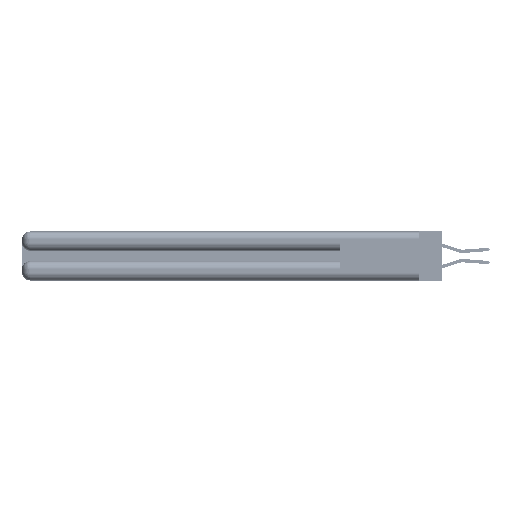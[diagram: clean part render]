
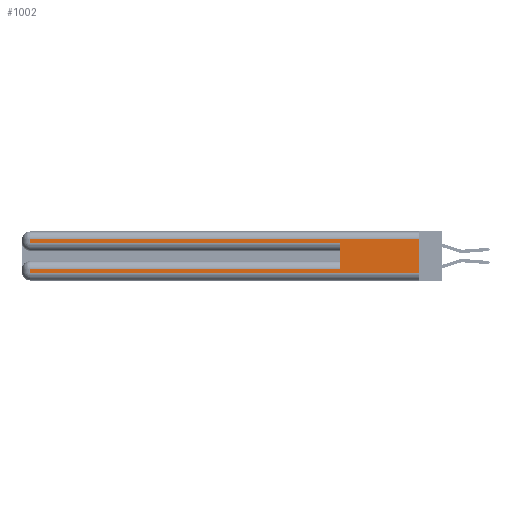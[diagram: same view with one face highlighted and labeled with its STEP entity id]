
A CAD part, left-side view. The second image highlights one B-rep face of the part: STEP entity #1002.
In plain terms, the highlighted planar face has unit normal (-1, 0, 0).
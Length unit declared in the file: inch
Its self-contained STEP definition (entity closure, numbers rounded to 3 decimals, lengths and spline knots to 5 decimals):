
#523 = VERTEX_POINT ( 'NONE', #30071 ) ;
#1002 = ADVANCED_FACE ( 'NONE', ( #9338 ), #17285, .F. ) ;
#1548 = LINE ( 'NONE', #7490, #26952 ) ;
#1995 = VERTEX_POINT ( 'NONE', #23235 ) ;
#3073 = CARTESIAN_POINT ( 'NONE',  ( 0., 0., 0.06 ) ) ;
#4491 = VERTEX_POINT ( 'NONE', #18902 ) ;
#4835 = DIRECTION ( 'NONE',  ( 0., 0., -1. ) ) ;
#7236 = ORIENTED_EDGE ( 'NONE', *, *, #49218, .F. ) ;
#7490 = CARTESIAN_POINT ( 'NONE',  ( 0., 2.94, 0.37 ) ) ;
#7836 = VERTEX_POINT ( 'NONE', #25975 ) ;
#7871 = ORIENTED_EDGE ( 'NONE', *, *, #21200, .T. ) ;
#9338 = FACE_OUTER_BOUND ( 'NONE', #22766, .T. ) ;
#10640 = LINE ( 'NONE', #19429, #52046 ) ;
#12660 = VERTEX_POINT ( 'NONE', #15950 ) ;
#12858 = EDGE_CURVE ( 'NONE', #4491, #7836, #22673, .T. ) ;
#12895 = VECTOR ( 'NONE', #53563, 39.37008 ) ;
#12971 = EDGE_CURVE ( 'NONE', #28785, #523, #10640, .T. ) ;
#14642 = VECTOR ( 'NONE', #39849, 39.37008 ) ;
#15042 = VERTEX_POINT ( 'NONE', #37919 ) ;
#15338 = CARTESIAN_POINT ( 'NONE',  ( 0., 0.6, 0.085 ) ) ;
#15950 = CARTESIAN_POINT ( 'NONE',  ( 0., 2.94, 0.285 ) ) ;
#16309 = EDGE_CURVE ( 'NONE', #15042, #49202, #18681, .T. ) ;
#17285 = PLANE ( 'NONE',  #29171 ) ;
#17325 = ORIENTED_EDGE ( 'NONE', *, *, #37101, .T. ) ;
#18002 = LINE ( 'NONE', #53822, #53384 ) ;
#18681 = LINE ( 'NONE', #3073, #41438 ) ;
#18902 = CARTESIAN_POINT ( 'NONE',  ( 0., 0., 0.31 ) ) ;
#19429 = CARTESIAN_POINT ( 'NONE',  ( 0., 0.6, 0.145 ) ) ;
#19530 = DIRECTION ( 'NONE',  ( 0., -1., 0. ) ) ;
#20743 = DIRECTION ( 'NONE',  ( 0., -1., 0. ) ) ;
#21200 = EDGE_CURVE ( 'NONE', #28785, #1995, #24254, .T. ) ;
#22089 = CARTESIAN_POINT ( 'NONE',  ( 0., 0., 0.31 ) ) ;
#22673 = LINE ( 'NONE', #22089, #14642 ) ;
#22766 = EDGE_LOOP ( 'NONE', ( #7236, #30503, #51929, #17325, #30945, #7871, #30995, #26364 ) ) ;
#23235 = CARTESIAN_POINT ( 'NONE',  ( 0., 2.94, 0.085 ) ) ;
#23331 = VECTOR ( 'NONE', #4835, 39.37008 ) ;
#24254 = LINE ( 'NONE', #44997, #12895 ) ;
#25679 = LINE ( 'NONE', #41418, #26386 ) ;
#25975 = CARTESIAN_POINT ( 'NONE',  ( 0., 2.94, 0.31 ) ) ;
#26028 = LINE ( 'NONE', #30062, #23331 ) ;
#26364 = ORIENTED_EDGE ( 'NONE', *, *, #16309, .T. ) ;
#26386 = VECTOR ( 'NONE', #19530, 39.37008 ) ;
#26952 = VECTOR ( 'NONE', #38095, 39.37008 ) ;
#28785 = VERTEX_POINT ( 'NONE', #15338 ) ;
#28950 = EDGE_CURVE ( 'NONE', #1995, #15042, #1548, .T. ) ;
#29171 = AXIS2_PLACEMENT_3D ( 'NONE', #34512, #38614, #47177 ) ;
#30062 = CARTESIAN_POINT ( 'NONE',  ( 0., 2.94, 0.37 ) ) ;
#30071 = CARTESIAN_POINT ( 'NONE',  ( 0., 0.6, 0.285 ) ) ;
#30503 = ORIENTED_EDGE ( 'NONE', *, *, #12858, .T. ) ;
#30945 = ORIENTED_EDGE ( 'NONE', *, *, #12971, .F. ) ;
#30995 = ORIENTED_EDGE ( 'NONE', *, *, #28950, .T. ) ;
#34512 = CARTESIAN_POINT ( 'NONE',  ( 0., 0., 0.37 ) ) ;
#37101 = EDGE_CURVE ( 'NONE', #12660, #523, #25679, .T. ) ;
#37408 = CARTESIAN_POINT ( 'NONE',  ( 0., 0., 0.06 ) ) ;
#37919 = CARTESIAN_POINT ( 'NONE',  ( 0., 2.94, 0.06 ) ) ;
#38095 = DIRECTION ( 'NONE',  ( 0., 0., -1. ) ) ;
#38614 = DIRECTION ( 'NONE',  ( 1., 0., 0. ) ) ;
#39849 = DIRECTION ( 'NONE',  ( 0., 1., 0. ) ) ;
#41146 = DIRECTION ( 'NONE',  ( 0., 0., -1. ) ) ;
#41418 = CARTESIAN_POINT ( 'NONE',  ( 0., 0., 0.285 ) ) ;
#41438 = VECTOR ( 'NONE', #20743, 39.37008 ) ;
#44997 = CARTESIAN_POINT ( 'NONE',  ( 0., 0., 0.085 ) ) ;
#47177 = DIRECTION ( 'NONE',  ( 0., 0., -1. ) ) ;
#48760 = DIRECTION ( 'NONE',  ( 0., 0., 1. ) ) ;
#49202 = VERTEX_POINT ( 'NONE', #37408 ) ;
#49218 = EDGE_CURVE ( 'NONE', #4491, #49202, #18002, .T. ) ;
#51929 = ORIENTED_EDGE ( 'NONE', *, *, #54754, .T. ) ;
#52046 = VECTOR ( 'NONE', #48760, 39.37008 ) ;
#53384 = VECTOR ( 'NONE', #41146, 39.37008 ) ;
#53563 = DIRECTION ( 'NONE',  ( 0., 1., 0. ) ) ;
#53822 = CARTESIAN_POINT ( 'NONE',  ( 0., 0., 0.37 ) ) ;
#54754 = EDGE_CURVE ( 'NONE', #7836, #12660, #26028, .T. ) ;
